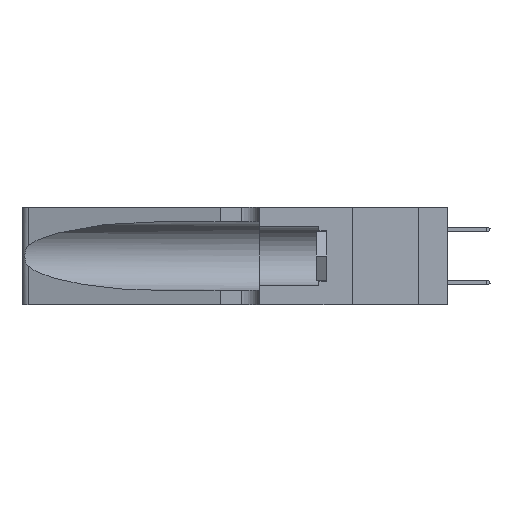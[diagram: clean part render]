
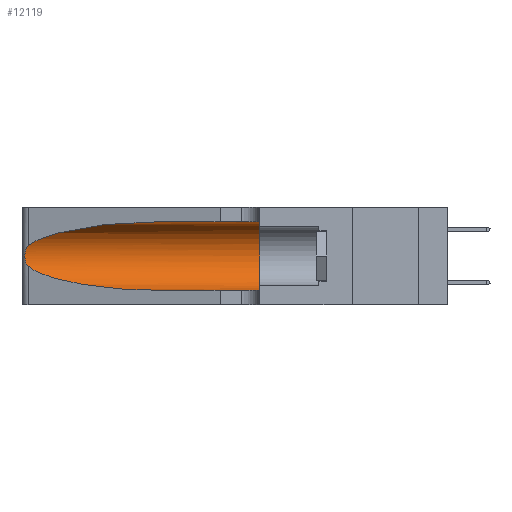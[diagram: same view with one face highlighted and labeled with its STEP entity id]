
A CAD part, left-side view. The second image highlights one B-rep face of the part: STEP entity #12119.
In plain terms, the highlighted cylindrical face has radius 3.308 mm (diameter 6.617 mm), a partial arc.
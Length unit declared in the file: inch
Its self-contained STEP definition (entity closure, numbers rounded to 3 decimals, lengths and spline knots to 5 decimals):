
#1103 = CARTESIAN_POINT ( 'NONE',  ( 0.1305, 1.61858, 0.05475 ) ) ;
#1281 = VERTEX_POINT ( 'NONE', #6886 ) ;
#2182 = CARTESIAN_POINT ( 'NONE',  ( 0.26018, 1.23835, 0.19895 ) ) ;
#2254 = CIRCLE ( 'NONE', #35233, 0.13025 ) ;
#2453 = ORIENTED_EDGE ( 'NONE', *, *, #20757, .T. ) ;
#2754 = DIRECTION ( 'NONE',  ( 0., 1., 0. ) ) ;
#3116 = DIRECTION ( 'NONE',  ( 0., 0., -1. ) ) ;
#4197 = ORIENTED_EDGE ( 'NONE', *, *, #12018, .F. ) ;
#4434 = EDGE_CURVE ( 'NONE', #16166, #32732, #13863, .T. ) ;
#4603 = CARTESIAN_POINT ( 'NONE',  ( 0.18966, 0.96281, 0.05475 ) ) ;
#4877 = DIRECTION ( 'NONE',  ( 0., -1., 0. ) ) ;
#4999 = CARTESIAN_POINT ( 'NONE',  ( 0.26075, 1.23896, 0.178 ) ) ;
#5317 = CARTESIAN_POINT ( 'NONE',  ( 0.1305, 0.72297, 0.05475 ) ) ;
#5495 = ORIENTED_EDGE ( 'NONE', *, *, #4434, .T. ) ;
#6154 = VERTEX_POINT ( 'NONE', #17668 ) ;
#6161 = CARTESIAN_POINT ( 'NONE',  ( 0.1305, 0.35, 0.31525 ) ) ;
#6453 = LINE ( 'NONE', #1103, #34505 ) ;
#6886 = CARTESIAN_POINT ( 'NONE',  ( 0.1305, 0.72297, 0.31525 ) ) ;
#7732 = CARTESIAN_POINT ( 'NONE',  ( 0.25856, 1.23593, 0.16098 ) ) ;
#8230 = VECTOR ( 'NONE', #4877, 39.37008 ) ;
#10046 = CARTESIAN_POINT ( 'NONE',  ( 0.25487, 1.22718, 0.14631 ) ) ;
#10430 = CARTESIAN_POINT ( 'NONE',  ( 0.1305, 1.61858, 0.31525 ) ) ;
#10548 = CARTESIAN_POINT ( 'NONE',  ( 0.25639, 1.23186, 0.15144 ) ) ;
#11566 = ORIENTED_EDGE ( 'NONE', *, *, #13239, .F. ) ;
#12018 = EDGE_CURVE ( 'NONE', #21874, #6154, #2254, .T. ) ;
#12119 = ADVANCED_FACE ( 'NONE', ( #20727 ), #22885, .F. ) ;
#13209 = CARTESIAN_POINT ( 'NONE',  ( 0.25639, 1.23184, 0.21858 ) ) ;
#13239 = EDGE_CURVE ( 'NONE', #1281, #21874, #29937, .T. ) ;
#13317 = CARTESIAN_POINT ( 'NONE',  ( 0.25487, 1.22718, 0.14631 ) ) ;
#13863 = B_SPLINE_CURVE_WITH_KNOTS ( 'NONE', 3,
 ( #29413, #32097, #13209, #34811, #18668, #2182, #21397, #4999, #24109, #7732, #26817, #10548, #29531, #13317 ),
 .UNSPECIFIED., .F., .F.,
 ( 4, 2, 2, 2, 2, 2, 4 ),
 ( 0., 0.00027, 0.00053, 0.00107, 0.0016, 0.00187, 0.00214 ),
 .UNSPECIFIED. ) ;
#13905 = VERTEX_POINT ( 'NONE', #5317 ) ;
#14684 = AXIS2_PLACEMENT_3D ( 'NONE', #22299, #25007, #3116 ) ;
#14974 = ORIENTED_EDGE ( 'NONE', *, *, #28609, .T. ) ;
#16166 = VERTEX_POINT ( 'NONE', #27962 ) ;
#17668 = CARTESIAN_POINT ( 'NONE',  ( 0.1305, 0.35, 0.05475 ) ) ;
#18288 = CARTESIAN_POINT ( 'NONE',  ( 0.25487, 1.22718, 0.14631 ) ) ;
#18668 = CARTESIAN_POINT ( 'NONE',  ( 0.25854, 1.2359, 0.20912 ) ) ;
#18843 = CARTESIAN_POINT ( 'NONE',  ( 0.25487, 1.22718, 0.22369 ) ) ;
#19214 = CARTESIAN_POINT ( 'NONE',  ( 0.1305, 0.35, 0.185 ) ) ;
#20727 = FACE_OUTER_BOUND ( 'NONE', #31543, .T. ) ;
#20757 = EDGE_CURVE ( 'NONE', #13905, #6154, #6453, .T. ) ;
#20908 = ORIENTED_EDGE ( 'NONE', *, *, #32734, .T. ) ;
#21264 =( BOUNDED_CURVE ( )  B_SPLINE_CURVE ( 3, ( #18288, #26327, #4603, #23746 ),
 .UNSPECIFIED., .F., .T. ) 
 B_SPLINE_CURVE_WITH_KNOTS ( ( 4, 4 ),
 ( 3.44316, 4.71239 ),
 .UNSPECIFIED. ) 
 CURVE ( )  GEOMETRIC_REPRESENTATION_ITEM ( )  RATIONAL_B_SPLINE_CURVE ( ( 1., 0.87, 0.87, 1. ) ) 
 REPRESENTATION_ITEM ( '' )  );
#21397 = CARTESIAN_POINT ( 'NONE',  ( 0.26075, 1.23896, 0.19203 ) ) ;
#21874 = VERTEX_POINT ( 'NONE', #6161 ) ;
#21937 = DIRECTION ( 'NONE',  ( 0., 0., 1. ) ) ;
#22299 = CARTESIAN_POINT ( 'NONE',  ( 0.1305, 1.61858, 0.185 ) ) ;
#22885 = CYLINDRICAL_SURFACE ( 'NONE', #14684, 0.13025 ) ;
#23746 = CARTESIAN_POINT ( 'NONE',  ( 0.1305, 0.72297, 0.05475 ) ) ;
#24109 = CARTESIAN_POINT ( 'NONE',  ( 0.26017, 1.23833, 0.17102 ) ) ;
#25007 = DIRECTION ( 'NONE',  ( 0., -1., 0. ) ) ;
#26327 = CARTESIAN_POINT ( 'NONE',  ( 0.2373, 1.15595, 0.08982 ) ) ;
#26817 = CARTESIAN_POINT ( 'NONE',  ( 0.25789, 1.23486, 0.15765 ) ) ;
#27962 = CARTESIAN_POINT ( 'NONE',  ( 0.25487, 1.22718, 0.22369 ) ) ;
#28609 = EDGE_CURVE ( 'NONE', #1281, #16166, #33782, .T. ) ;
#29413 = CARTESIAN_POINT ( 'NONE',  ( 0.25487, 1.22718, 0.22369 ) ) ;
#29531 = CARTESIAN_POINT ( 'NONE',  ( 0.25555, 1.22993, 0.14849 ) ) ;
#29589 = CARTESIAN_POINT ( 'NONE',  ( 0.18966, 0.96281, 0.31525 ) ) ;
#29937 = LINE ( 'NONE', #10430, #8230 ) ;
#31199 = DIRECTION ( 'NONE',  ( 0., -1., 0. ) ) ;
#31543 = EDGE_LOOP ( 'NONE', ( #14974, #5495, #20908, #2453, #4197, #11566 ) ) ;
#32097 = CARTESIAN_POINT ( 'NONE',  ( 0.25555, 1.22994, 0.2215 ) ) ;
#32277 = CARTESIAN_POINT ( 'NONE',  ( 0.1305, 0.72297, 0.31525 ) ) ;
#32732 = VERTEX_POINT ( 'NONE', #10046 ) ;
#32734 = EDGE_CURVE ( 'NONE', #32732, #13905, #21264, .T. ) ;
#33782 =( BOUNDED_CURVE ( )  B_SPLINE_CURVE ( 3, ( #32277, #29589, #34984, #18843 ),
 .UNSPECIFIED., .F., .F. ) 
 B_SPLINE_CURVE_WITH_KNOTS ( ( 4, 4 ),
 ( 1.5708, 2.84003 ),
 .UNSPECIFIED. ) 
 CURVE ( )  GEOMETRIC_REPRESENTATION_ITEM ( )  RATIONAL_B_SPLINE_CURVE ( ( 1., 0.87, 0.87, 1. ) ) 
 REPRESENTATION_ITEM ( '' )  );
#34505 = VECTOR ( 'NONE', #31199, 39.37008 ) ;
#34811 = CARTESIAN_POINT ( 'NONE',  ( 0.25787, 1.23484, 0.2124 ) ) ;
#34984 = CARTESIAN_POINT ( 'NONE',  ( 0.2373, 1.15595, 0.28018 ) ) ;
#35233 = AXIS2_PLACEMENT_3D ( 'NONE', #19214, #2754, #21937 ) ;
